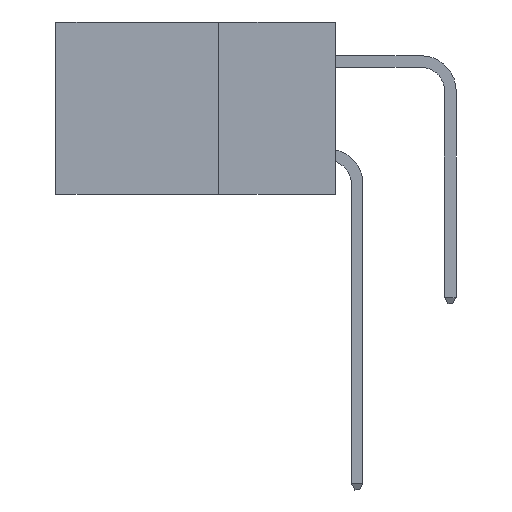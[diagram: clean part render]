
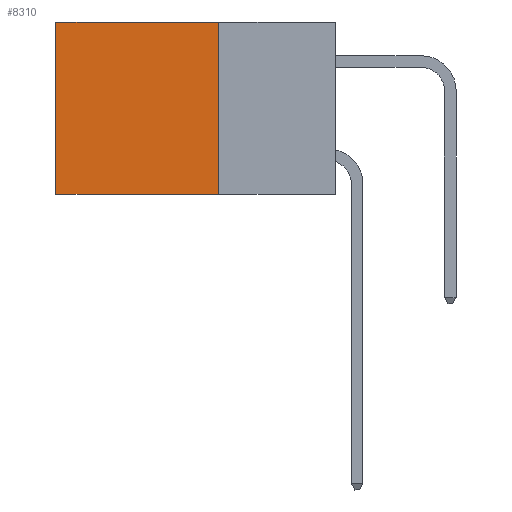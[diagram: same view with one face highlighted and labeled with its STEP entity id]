
A CAD part, left-side view. The second image highlights one B-rep face of the part: STEP entity #8310.
In plain terms, the highlighted planar face has unit normal (-1, 0, 0).
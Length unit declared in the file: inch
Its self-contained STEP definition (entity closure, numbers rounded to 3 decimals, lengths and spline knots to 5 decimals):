
#2066 = LINE ( 'NONE', #11913, #31980 ) ;
#3601 = EDGE_CURVE ( 'NONE', #13318, #23268, #31549, .T. ) ;
#5571 = ORIENTED_EDGE ( 'NONE', *, *, #33377, .T. ) ;
#8190 = DIRECTION ( 'NONE',  ( 0., 1., 0. ) ) ;
#8310 = ADVANCED_FACE ( 'NONE', ( #23825 ), #20613, .F. ) ;
#9157 = VECTOR ( 'NONE', #11838, 39.37008 ) ;
#11109 = DIRECTION ( 'NONE',  ( 0., 0., -1. ) ) ;
#11712 = CARTESIAN_POINT ( 'NONE',  ( 0.2875, 0.25, 0. ) ) ;
#11838 = DIRECTION ( 'NONE',  ( 0., 0., -1. ) ) ;
#11913 = CARTESIAN_POINT ( 'NONE',  ( 0.2875, 0.25, -0.37 ) ) ;
#13318 = VERTEX_POINT ( 'NONE', #28880 ) ;
#13754 = CARTESIAN_POINT ( 'NONE',  ( 0.2875, 0.25, 0. ) ) ;
#14938 = VERTEX_POINT ( 'NONE', #30407 ) ;
#14986 = EDGE_CURVE ( 'NONE', #13318, #35909, #34339, .T. ) ;
#15086 = DIRECTION ( 'NONE',  ( 1., 0., 0. ) ) ;
#15450 = CARTESIAN_POINT ( 'NONE',  ( 0.2875, 0.6, 0. ) ) ;
#18481 = ORIENTED_EDGE ( 'NONE', *, *, #3601, .F. ) ;
#19529 = CARTESIAN_POINT ( 'NONE',  ( 0.2875, 0.6, 0. ) ) ;
#20389 = AXIS2_PLACEMENT_3D ( 'NONE', #31829, #15086, #34631 ) ;
#20613 = PLANE ( 'NONE',  #20389 ) ;
#20740 = EDGE_LOOP ( 'NONE', ( #5571, #26605, #18481, #24752 ) ) ;
#23268 = VERTEX_POINT ( 'NONE', #34737 ) ;
#23825 = FACE_OUTER_BOUND ( 'NONE', #20740, .T. ) ;
#24752 = ORIENTED_EDGE ( 'NONE', *, *, #14986, .T. ) ;
#26605 = ORIENTED_EDGE ( 'NONE', *, *, #35034, .F. ) ;
#26919 = VECTOR ( 'NONE', #8190, 39.37008 ) ;
#28880 = CARTESIAN_POINT ( 'NONE',  ( 0.2875, 0.25, 0. ) ) ;
#30407 = CARTESIAN_POINT ( 'NONE',  ( 0.2875, 0.6, -0.37 ) ) ;
#31378 = VECTOR ( 'NONE', #11109, 39.37008 ) ;
#31531 = DIRECTION ( 'NONE',  ( 0., 1., 0. ) ) ;
#31549 = LINE ( 'NONE', #11712, #9157 ) ;
#31829 = CARTESIAN_POINT ( 'NONE',  ( 0.2875, 0.25, 0. ) ) ;
#31980 = VECTOR ( 'NONE', #31531, 39.37008 ) ;
#33377 = EDGE_CURVE ( 'NONE', #35909, #14938, #34866, .T. ) ;
#34339 = LINE ( 'NONE', #13754, #26919 ) ;
#34631 = DIRECTION ( 'NONE',  ( 0., 0., -1. ) ) ;
#34737 = CARTESIAN_POINT ( 'NONE',  ( 0.2875, 0.25, -0.37 ) ) ;
#34866 = LINE ( 'NONE', #19529, #31378 ) ;
#35034 = EDGE_CURVE ( 'NONE', #23268, #14938, #2066, .T. ) ;
#35909 = VERTEX_POINT ( 'NONE', #15450 ) ;
